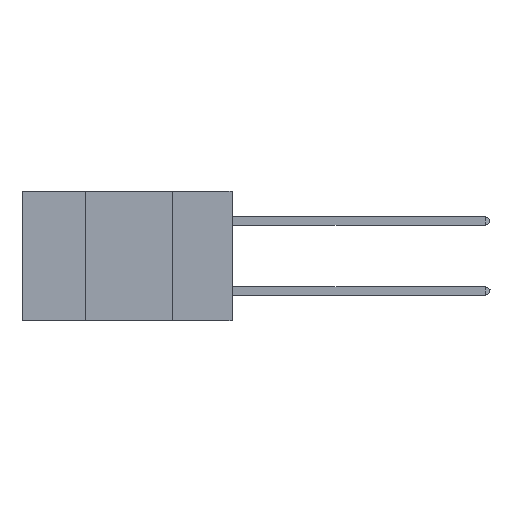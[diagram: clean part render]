
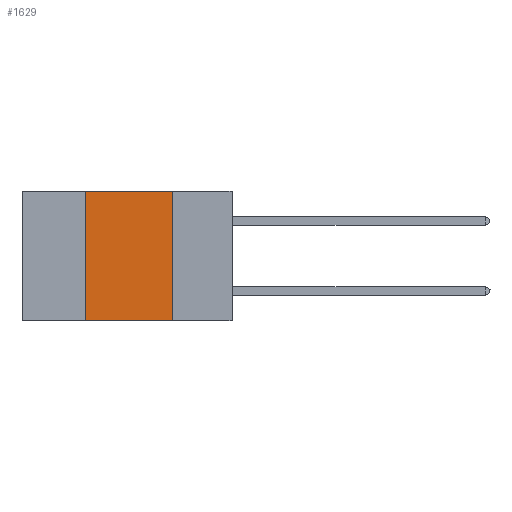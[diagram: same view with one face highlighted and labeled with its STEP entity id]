
A CAD part, left-side view. The second image highlights one B-rep face of the part: STEP entity #1629.
In plain terms, the highlighted planar face has unit normal (-1, 0, 0).
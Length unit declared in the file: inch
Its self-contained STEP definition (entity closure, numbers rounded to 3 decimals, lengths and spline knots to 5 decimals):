
#224 = DIRECTION ( 'NONE',  ( 0., 0., -1. ) ) ;
#454 = VERTEX_POINT ( 'NONE', #3790 ) ;
#568 = CARTESIAN_POINT ( 'NONE',  ( 0., 0.6, 0. ) ) ;
#607 = AXIS2_PLACEMENT_3D ( 'NONE', #2791, #10634, #224 ) ;
#1265 = CARTESIAN_POINT ( 'NONE',  ( 0., 0.17, 0. ) ) ;
#1580 = ORIENTED_EDGE ( 'NONE', *, *, #7612, .F. ) ;
#1629 = ADVANCED_FACE ( 'NONE', ( #9686 ), #11409, .F. ) ;
#1697 = DIRECTION ( 'NONE',  ( 0., 0., 1. ) ) ;
#1868 = VECTOR ( 'NONE', #10568, 39.37008 ) ;
#2791 = CARTESIAN_POINT ( 'NONE',  ( 0., 0.6, 0. ) ) ;
#2853 = ORIENTED_EDGE ( 'NONE', *, *, #11957, .F. ) ;
#3061 = EDGE_LOOP ( 'NONE', ( #2853, #1580, #3883, #10757 ) ) ;
#3208 = CARTESIAN_POINT ( 'NONE',  ( 0., 0.17, 0. ) ) ;
#3588 = EDGE_CURVE ( 'NONE', #454, #11082, #7085, .T. ) ;
#3790 = CARTESIAN_POINT ( 'NONE',  ( 0., 0.42, -0.37 ) ) ;
#3877 = VECTOR ( 'NONE', #7769, 39.37008 ) ;
#3883 = ORIENTED_EDGE ( 'NONE', *, *, #8524, .F. ) ;
#4675 = VERTEX_POINT ( 'NONE', #10900 ) ;
#5133 = VECTOR ( 'NONE', #1697, 39.37008 ) ;
#6927 = CARTESIAN_POINT ( 'NONE',  ( 0., 0.6, -0.37 ) ) ;
#7085 = LINE ( 'NONE', #6927, #3877 ) ;
#7612 = EDGE_CURVE ( 'NONE', #4675, #11112, #10595, .T. ) ;
#7624 = CARTESIAN_POINT ( 'NONE',  ( 0., 0.17, -0.37 ) ) ;
#7769 = DIRECTION ( 'NONE',  ( 0., -1., 0. ) ) ;
#8524 = EDGE_CURVE ( 'NONE', #454, #4675, #10321, .T. ) ;
#9310 = VECTOR ( 'NONE', #10141, 39.37008 ) ;
#9686 = FACE_OUTER_BOUND ( 'NONE', #3061, .T. ) ;
#10141 = DIRECTION ( 'NONE',  ( 0., -1., 0. ) ) ;
#10321 = LINE ( 'NONE', #10322, #5133 ) ;
#10322 = CARTESIAN_POINT ( 'NONE',  ( 0., 0.42, 0. ) ) ;
#10568 = DIRECTION ( 'NONE',  ( 0., 0., -1. ) ) ;
#10595 = LINE ( 'NONE', #568, #9310 ) ;
#10634 = DIRECTION ( 'NONE',  ( 1., 0., 0. ) ) ;
#10757 = ORIENTED_EDGE ( 'NONE', *, *, #3588, .T. ) ;
#10900 = CARTESIAN_POINT ( 'NONE',  ( 0., 0.42, 0. ) ) ;
#11082 = VERTEX_POINT ( 'NONE', #7624 ) ;
#11112 = VERTEX_POINT ( 'NONE', #1265 ) ;
#11409 = PLANE ( 'NONE',  #607 ) ;
#11957 = EDGE_CURVE ( 'NONE', #11112, #11082, #12108, .T. ) ;
#12108 = LINE ( 'NONE', #3208, #1868 ) ;
